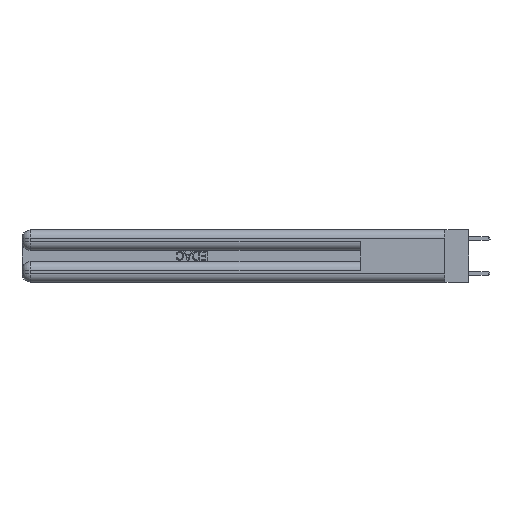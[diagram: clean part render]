
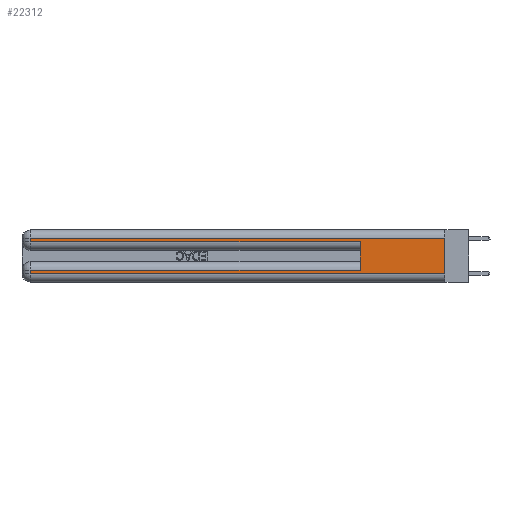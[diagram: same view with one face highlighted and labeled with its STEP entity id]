
A CAD part, left-side view. The second image highlights one B-rep face of the part: STEP entity #22312.
In plain terms, the highlighted planar face has unit normal (-1, 0, 0).
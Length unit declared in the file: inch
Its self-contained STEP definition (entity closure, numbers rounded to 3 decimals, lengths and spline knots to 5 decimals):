
#8 = ORIENTED_EDGE ( 'NONE', *, *, #28899, .T. ) ;
#1868 = LINE ( 'NONE', #11474, #27776 ) ;
#4448 = DIRECTION ( 'NONE',  ( 0., -1., 0. ) ) ;
#5026 = EDGE_CURVE ( 'NONE', #27525, #10140, #31905, .T. ) ;
#5412 = EDGE_CURVE ( 'NONE', #18422, #6073, #19148, .T. ) ;
#5914 = VECTOR ( 'NONE', #9272, 39.37008 ) ;
#5950 = FACE_OUTER_BOUND ( 'NONE', #16469, .T. ) ;
#6073 = VERTEX_POINT ( 'NONE', #20904 ) ;
#6780 = CARTESIAN_POINT ( 'NONE',  ( 0., 0., 0.06 ) ) ;
#7342 = CARTESIAN_POINT ( 'NONE',  ( 0., 0.6, 0.145 ) ) ;
#7945 = EDGE_CURVE ( 'NONE', #10343, #11515, #13596, .T. ) ;
#7984 = EDGE_CURVE ( 'NONE', #11826, #26935, #11750, .T. ) ;
#9196 = ORIENTED_EDGE ( 'NONE', *, *, #5026, .T. ) ;
#9218 = CARTESIAN_POINT ( 'NONE',  ( 0., 0., 0.085 ) ) ;
#9255 = CARTESIAN_POINT ( 'NONE',  ( 0., 0., 0.06 ) ) ;
#9269 = CARTESIAN_POINT ( 'NONE',  ( 0., 2.94, 0.06 ) ) ;
#9272 = DIRECTION ( 'NONE',  ( 0., 1., 0. ) ) ;
#9421 = ORIENTED_EDGE ( 'NONE', *, *, #25013, .F. ) ;
#9819 = EDGE_CURVE ( 'NONE', #18422, #11515, #17442, .T. ) ;
#10140 = VERTEX_POINT ( 'NONE', #6780 ) ;
#10343 = VERTEX_POINT ( 'NONE', #15055 ) ;
#10604 = VECTOR ( 'NONE', #32470, 39.37008 ) ;
#11133 = VECTOR ( 'NONE', #4448, 39.37008 ) ;
#11230 = CARTESIAN_POINT ( 'NONE',  ( 0., 0., 0.37 ) ) ;
#11474 = CARTESIAN_POINT ( 'NONE',  ( 0., 2.94, 0.37 ) ) ;
#11515 = VERTEX_POINT ( 'NONE', #24035 ) ;
#11750 = LINE ( 'NONE', #16892, #5914 ) ;
#11826 = VERTEX_POINT ( 'NONE', #14078 ) ;
#11919 = LINE ( 'NONE', #27294, #20571 ) ;
#12206 = CARTESIAN_POINT ( 'NONE',  ( 0., 0., 0.37 ) ) ;
#13596 = LINE ( 'NONE', #26651, #24917 ) ;
#13806 = DIRECTION ( 'NONE',  ( 0., 0., -1. ) ) ;
#14078 = CARTESIAN_POINT ( 'NONE',  ( 0., 0., 0.31 ) ) ;
#14213 = LINE ( 'NONE', #12206, #27794 ) ;
#15055 = CARTESIAN_POINT ( 'NONE',  ( 0., 2.94, 0.285 ) ) ;
#16056 = DIRECTION ( 'NONE',  ( 0., 0., -1. ) ) ;
#16240 = ORIENTED_EDGE ( 'NONE', *, *, #9819, .F. ) ;
#16469 = EDGE_LOOP ( 'NONE', ( #9421, #27469, #8, #19573, #16240, #31974, #21402, #9196 ) ) ;
#16703 = DIRECTION ( 'NONE',  ( 0., 0., -1. ) ) ;
#16892 = CARTESIAN_POINT ( 'NONE',  ( 0., 0., 0.31 ) ) ;
#16997 = CARTESIAN_POINT ( 'NONE',  ( 0., 0.6, 0.085 ) ) ;
#17442 = LINE ( 'NONE', #7342, #10604 ) ;
#18197 = PLANE ( 'NONE',  #30402 ) ;
#18422 = VERTEX_POINT ( 'NONE', #16997 ) ;
#19148 = LINE ( 'NONE', #9218, #22749 ) ;
#19573 = ORIENTED_EDGE ( 'NONE', *, *, #7945, .T. ) ;
#20571 = VECTOR ( 'NONE', #27461, 39.37008 ) ;
#20904 = CARTESIAN_POINT ( 'NONE',  ( 0., 2.94, 0.085 ) ) ;
#21402 = ORIENTED_EDGE ( 'NONE', *, *, #24596, .T. ) ;
#21718 = CARTESIAN_POINT ( 'NONE',  ( 0., 2.94, 0.31 ) ) ;
#22312 = ADVANCED_FACE ( 'NONE', ( #5950 ), #18197, .F. ) ;
#22749 = VECTOR ( 'NONE', #23953, 39.37008 ) ;
#23953 = DIRECTION ( 'NONE',  ( 0., 1., 0. ) ) ;
#24035 = CARTESIAN_POINT ( 'NONE',  ( 0., 0.6, 0.285 ) ) ;
#24596 = EDGE_CURVE ( 'NONE', #6073, #27525, #1868, .T. ) ;
#24917 = VECTOR ( 'NONE', #26331, 39.37008 ) ;
#25013 = EDGE_CURVE ( 'NONE', #11826, #10140, #14213, .T. ) ;
#26331 = DIRECTION ( 'NONE',  ( 0., -1., 0. ) ) ;
#26651 = CARTESIAN_POINT ( 'NONE',  ( 0., 0., 0.285 ) ) ;
#26935 = VERTEX_POINT ( 'NONE', #21718 ) ;
#27294 = CARTESIAN_POINT ( 'NONE',  ( 0., 2.94, 0.37 ) ) ;
#27461 = DIRECTION ( 'NONE',  ( 0., 0., -1. ) ) ;
#27469 = ORIENTED_EDGE ( 'NONE', *, *, #7984, .T. ) ;
#27525 = VERTEX_POINT ( 'NONE', #9269 ) ;
#27776 = VECTOR ( 'NONE', #13806, 39.37008 ) ;
#27794 = VECTOR ( 'NONE', #16703, 39.37008 ) ;
#28279 = DIRECTION ( 'NONE',  ( 1., 0., 0. ) ) ;
#28899 = EDGE_CURVE ( 'NONE', #26935, #10343, #11919, .T. ) ;
#30402 = AXIS2_PLACEMENT_3D ( 'NONE', #11230, #28279, #16056 ) ;
#31905 = LINE ( 'NONE', #9255, #11133 ) ;
#31974 = ORIENTED_EDGE ( 'NONE', *, *, #5412, .T. ) ;
#32470 = DIRECTION ( 'NONE',  ( 0., 0., 1. ) ) ;
